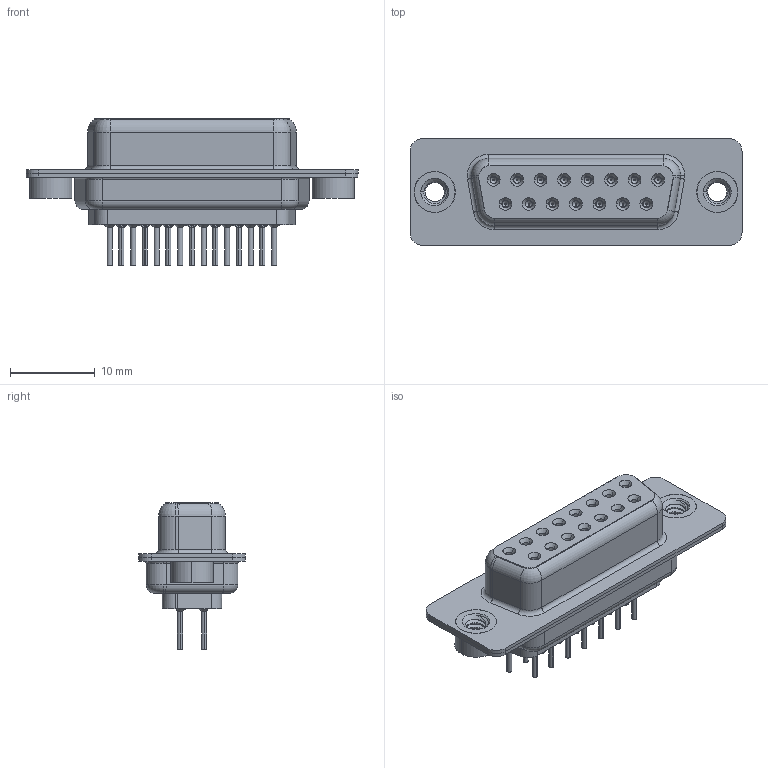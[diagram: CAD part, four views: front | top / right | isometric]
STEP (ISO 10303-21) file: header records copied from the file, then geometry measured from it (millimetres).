
FILE_DESCRIPTION (( 'STEP AP203' ), '1' );
FILE_NAME ('628-015-320-042.STEP', '2020-07-14T01:01:54', ( '' ), ( '' ), 'SwSTEP 2.0', 'SolidWorks 2020', '' );
FILE_SCHEMA (( 'CONFIG_CONTROL_DESIGN' ));
Length unit declared in the file: millimetre
Products named in the file (7): 628-015-320-042; 628 Shell Front_15 Contacts; 628 Contact Row 2_20L; 628 Contact Row 1_20L; 628 Housing_15 LP; 628 4-40 Threaded Rivet; 628 Shell Rear_15 Contacts
Assembly tree (20 placements, depth 2):
  628-015-320-042
    628 Housing_15 LP
    628 Shell Front_15 Contacts
    628 Shell Rear_15 Contacts
    628 Contact Row 1_20L  x8
    628 Contact Row 2_20L  x7
    628 4-40 Threaded Rivet  x2
Bounding box: 39.15 x 12.6 x 17.3 mm (x, y, z)
Volume: 2538.1 mm3; surface area: 6315 mm2
Topology: 20 solids, 20 shells, 2180 faces, 5535 edges, 3436 vertices
Faces by surface type: cylinder 630, plane 532, torus 447, bspline 306, cone 265
Entity records: 23959 total; most frequent: CARTESIAN_POINT 7305, DIRECTION 3374, ORIENTED_EDGE 3202, EDGE_CURVE 1601, AXIS2_PLACEMENT_3D 1403, VERTEX_POINT 1004, EDGE_LOOP 761, CIRCLE 760
